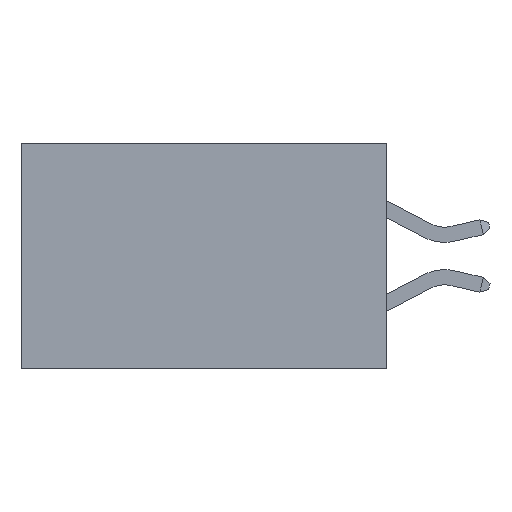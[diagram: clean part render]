
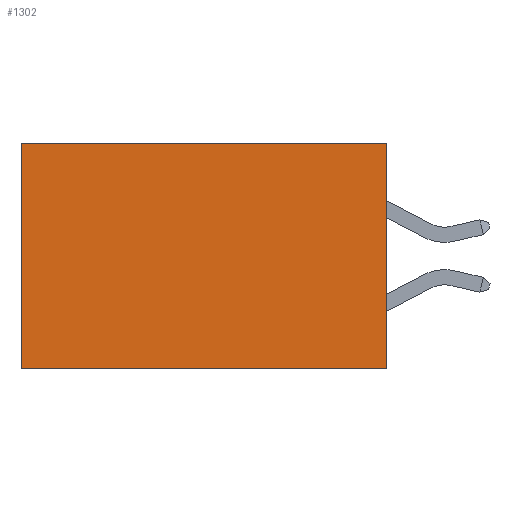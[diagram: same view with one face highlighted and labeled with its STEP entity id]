
A CAD part, left-side view. The second image highlights one B-rep face of the part: STEP entity #1302.
In plain terms, the highlighted planar face has unit normal (-1, 0, 0).
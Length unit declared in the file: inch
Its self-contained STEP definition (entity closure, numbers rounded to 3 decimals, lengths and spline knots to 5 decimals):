
#30 = VECTOR ( 'NONE', #8695, 39.37008 ) ;
#327 = LINE ( 'NONE', #8525, #30 ) ;
#400 = LINE ( 'NONE', #4234, #2132 ) ;
#506 = ORIENTED_EDGE ( 'NONE', *, *, #2078, .T. ) ;
#515 = AXIS2_PLACEMENT_3D ( 'NONE', #6992, #4535, #6818 ) ;
#1143 = LINE ( 'NONE', #6802, #4940 ) ;
#1302 = ADVANCED_FACE ( 'NONE', ( #7687 ), #7131, .F. ) ;
#1946 = CARTESIAN_POINT ( 'NONE',  ( 0.2615, 0., 0. ) ) ;
#2078 = EDGE_CURVE ( 'NONE', #8142, #6185, #327, .T. ) ;
#2132 = VECTOR ( 'NONE', #3700, 39.37008 ) ;
#2157 = DIRECTION ( 'NONE',  ( 0., 0., -1. ) ) ;
#2247 = CARTESIAN_POINT ( 'NONE',  ( 0.2615, 0., -0.37 ) ) ;
#2263 = EDGE_CURVE ( 'NONE', #6185, #6041, #1143, .T. ) ;
#2645 = ORIENTED_EDGE ( 'NONE', *, *, #2263, .T. ) ;
#3183 = EDGE_CURVE ( 'NONE', #7322, #6041, #400, .T. ) ;
#3211 = EDGE_CURVE ( 'NONE', #8142, #7322, #5496, .T. ) ;
#3700 = DIRECTION ( 'NONE',  ( 0., 1., 0. ) ) ;
#4022 = CARTESIAN_POINT ( 'NONE',  ( 0.2615, 0., -0.37 ) ) ;
#4144 = DIRECTION ( 'NONE',  ( 0., 0., -1. ) ) ;
#4234 = CARTESIAN_POINT ( 'NONE',  ( 0.2615, 0., -0.37 ) ) ;
#4535 = DIRECTION ( 'NONE',  ( 1., 0., 0. ) ) ;
#4940 = VECTOR ( 'NONE', #4144, 39.37008 ) ;
#5309 = VECTOR ( 'NONE', #2157, 39.37008 ) ;
#5496 = LINE ( 'NONE', #2247, #5309 ) ;
#6041 = VERTEX_POINT ( 'NONE', #6522 ) ;
#6185 = VERTEX_POINT ( 'NONE', #6330 ) ;
#6330 = CARTESIAN_POINT ( 'NONE',  ( 0.2615, 0.6, 0. ) ) ;
#6522 = CARTESIAN_POINT ( 'NONE',  ( 0.2615, 0.6, -0.37 ) ) ;
#6569 = ORIENTED_EDGE ( 'NONE', *, *, #3183, .F. ) ;
#6802 = CARTESIAN_POINT ( 'NONE',  ( 0.2615, 0.6, -0.37 ) ) ;
#6818 = DIRECTION ( 'NONE',  ( 0., 0., -1. ) ) ;
#6992 = CARTESIAN_POINT ( 'NONE',  ( 0.2615, 0., -0.37 ) ) ;
#7131 = PLANE ( 'NONE',  #515 ) ;
#7297 = ORIENTED_EDGE ( 'NONE', *, *, #3211, .F. ) ;
#7322 = VERTEX_POINT ( 'NONE', #4022 ) ;
#7687 = FACE_OUTER_BOUND ( 'NONE', #8269, .T. ) ;
#8142 = VERTEX_POINT ( 'NONE', #1946 ) ;
#8269 = EDGE_LOOP ( 'NONE', ( #2645, #6569, #7297, #506 ) ) ;
#8525 = CARTESIAN_POINT ( 'NONE',  ( 0.2615, 0., 0. ) ) ;
#8695 = DIRECTION ( 'NONE',  ( 0., 1., 0. ) ) ;
